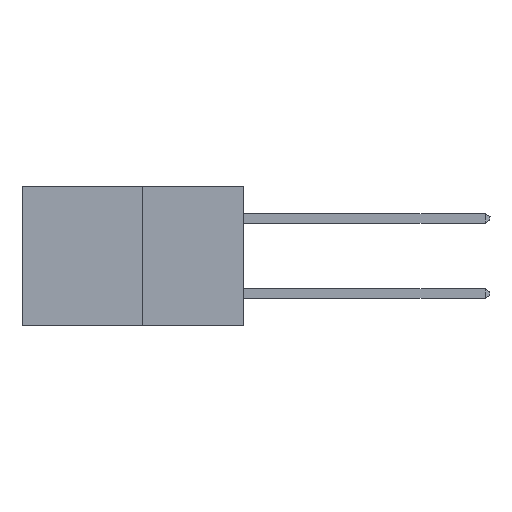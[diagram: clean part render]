
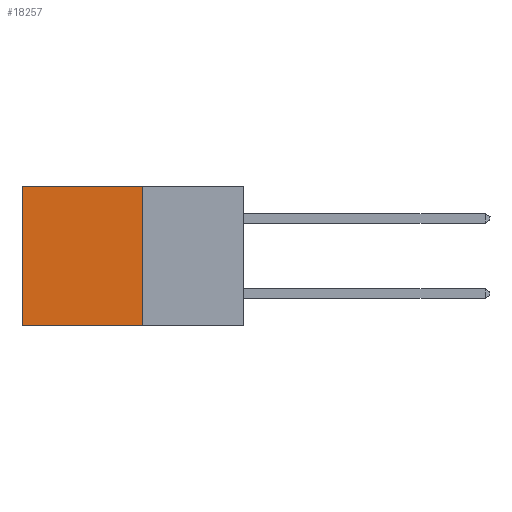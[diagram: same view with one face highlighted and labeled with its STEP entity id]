
A CAD part, left-side view. The second image highlights one B-rep face of the part: STEP entity #18257.
In plain terms, the highlighted planar face has unit normal (-1, 0, 0).
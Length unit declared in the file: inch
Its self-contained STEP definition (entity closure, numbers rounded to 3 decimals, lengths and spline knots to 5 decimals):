
#332 = CARTESIAN_POINT ( 'NONE',  ( 0.277, 0.27, -0.37 ) ) ;
#874 = EDGE_CURVE ( 'NONE', #23719, #12362, #23917, .T. ) ;
#1822 = CARTESIAN_POINT ( 'NONE',  ( 0.277, 0.59, -0.37 ) ) ;
#1967 = CARTESIAN_POINT ( 'NONE',  ( 0.277, 0.59, 0. ) ) ;
#1977 = CARTESIAN_POINT ( 'NONE',  ( 0.277, 0.27, -0.37 ) ) ;
#2631 = ORIENTED_EDGE ( 'NONE', *, *, #874, .T. ) ;
#4206 = DIRECTION ( 'NONE',  ( 0., 0., -1. ) ) ;
#5096 = DIRECTION ( 'NONE',  ( 0., 0., -1. ) ) ;
#5462 = DIRECTION ( 'NONE',  ( 0., 0., -1. ) ) ;
#5534 = CARTESIAN_POINT ( 'NONE',  ( 0.277, 0.59, -0.37 ) ) ;
#6040 = LINE ( 'NONE', #332, #23852 ) ;
#8081 = EDGE_LOOP ( 'NONE', ( #23669, #19721, #11101, #2631 ) ) ;
#8363 = VECTOR ( 'NONE', #4206, 39.37008 ) ;
#11101 = ORIENTED_EDGE ( 'NONE', *, *, #17645, .F. ) ;
#11783 = DIRECTION ( 'NONE',  ( 0., 1., 0. ) ) ;
#11969 = VERTEX_POINT ( 'NONE', #5534 ) ;
#12362 = VERTEX_POINT ( 'NONE', #1967 ) ;
#12454 = DIRECTION ( 'NONE',  ( 0., 1., 0. ) ) ;
#13895 = EDGE_CURVE ( 'NONE', #25008, #11969, #6040, .T. ) ;
#13986 = CARTESIAN_POINT ( 'NONE',  ( 0.277, 0.27, 0. ) ) ;
#17235 = PLANE ( 'NONE',  #24089 ) ;
#17645 = EDGE_CURVE ( 'NONE', #23719, #25008, #31118, .T. ) ;
#18257 = ADVANCED_FACE ( 'NONE', ( #27382 ), #17235, .F. ) ;
#19075 = VECTOR ( 'NONE', #5462, 39.37008 ) ;
#19643 = DIRECTION ( 'NONE',  ( 1., 0., 0. ) ) ;
#19721 = ORIENTED_EDGE ( 'NONE', *, *, #13895, .F. ) ;
#20007 = CARTESIAN_POINT ( 'NONE',  ( 0.277, 0.27, -0.37 ) ) ;
#23192 = VECTOR ( 'NONE', #11783, 39.37008 ) ;
#23669 = ORIENTED_EDGE ( 'NONE', *, *, #28632, .T. ) ;
#23719 = VERTEX_POINT ( 'NONE', #29081 ) ;
#23852 = VECTOR ( 'NONE', #12454, 39.37008 ) ;
#23917 = LINE ( 'NONE', #13986, #23192 ) ;
#24089 = AXIS2_PLACEMENT_3D ( 'NONE', #24386, #19643, #5096 ) ;
#24386 = CARTESIAN_POINT ( 'NONE',  ( 0.277, 0.27, -0.37 ) ) ;
#25008 = VERTEX_POINT ( 'NONE', #1977 ) ;
#27382 = FACE_OUTER_BOUND ( 'NONE', #8081, .T. ) ;
#27725 = LINE ( 'NONE', #1822, #8363 ) ;
#28632 = EDGE_CURVE ( 'NONE', #12362, #11969, #27725, .T. ) ;
#29081 = CARTESIAN_POINT ( 'NONE',  ( 0.277, 0.27, 0. ) ) ;
#31118 = LINE ( 'NONE', #20007, #19075 ) ;
